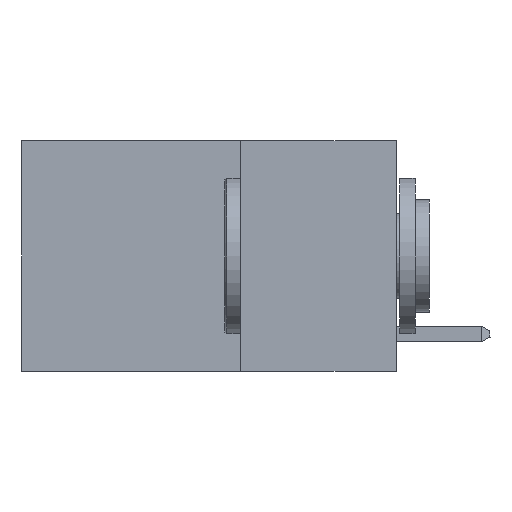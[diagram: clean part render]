
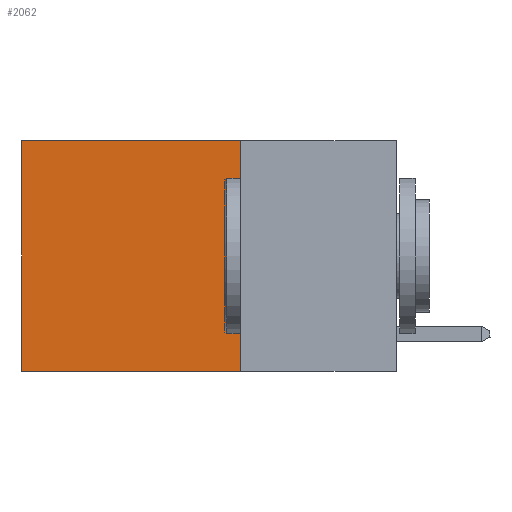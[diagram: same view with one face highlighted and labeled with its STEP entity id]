
A CAD part, left-side view. The second image highlights one B-rep face of the part: STEP entity #2062.
In plain terms, the highlighted planar face has unit normal (-1, 0, 0).
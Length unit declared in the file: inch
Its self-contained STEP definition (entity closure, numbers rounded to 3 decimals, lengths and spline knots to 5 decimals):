
#1244 = ORIENTED_EDGE ( 'NONE', *, *, #11885, .T. ) ;
#1545 = VECTOR ( 'NONE', #14747, 39.37008 ) ;
#1650 = DIRECTION ( 'NONE',  ( 0., 0., -1. ) ) ;
#1776 = CARTESIAN_POINT ( 'NONE',  ( 0.2625, 0.25, 0. ) ) ;
#2062 = ADVANCED_FACE ( 'NONE', ( #4222 ), #3379, .F. ) ;
#2165 = VERTEX_POINT ( 'NONE', #12706 ) ;
#2240 = EDGE_CURVE ( 'NONE', #9153, #14307, #15468, .T. ) ;
#2312 = DIRECTION ( 'NONE',  ( 1., 0., 0. ) ) ;
#2478 = DIRECTION ( 'NONE',  ( 0., 0., -1. ) ) ;
#2665 = LINE ( 'NONE', #5310, #6970 ) ;
#3100 = ORIENTED_EDGE ( 'NONE', *, *, #7772, .T. ) ;
#3379 = PLANE ( 'NONE',  #15404 ) ;
#3946 = ORIENTED_EDGE ( 'NONE', *, *, #2240, .F. ) ;
#4141 = CARTESIAN_POINT ( 'NONE',  ( 0.2625, 0.25, 0. ) ) ;
#4222 = FACE_OUTER_BOUND ( 'NONE', #15835, .T. ) ;
#5247 = CARTESIAN_POINT ( 'NONE',  ( 0.2625, 0.25, -0.37 ) ) ;
#5310 = CARTESIAN_POINT ( 'NONE',  ( 0.2625, 0.6, 0. ) ) ;
#6302 = VERTEX_POINT ( 'NONE', #1776 ) ;
#6707 = DIRECTION ( 'NONE',  ( 0., 1., 0. ) ) ;
#6970 = VECTOR ( 'NONE', #2478, 39.37008 ) ;
#7032 = CARTESIAN_POINT ( 'NONE',  ( 0.2625, 0.25, -0.37 ) ) ;
#7256 = CARTESIAN_POINT ( 'NONE',  ( 0.2625, 0.25, 0. ) ) ;
#7772 = EDGE_CURVE ( 'NONE', #6302, #2165, #15935, .T. ) ;
#8689 = DIRECTION ( 'NONE',  ( 0., 0., -1. ) ) ;
#8755 = VECTOR ( 'NONE', #6707, 39.37008 ) ;
#9116 = LINE ( 'NONE', #7256, #15828 ) ;
#9153 = VERTEX_POINT ( 'NONE', #5247 ) ;
#9398 = CARTESIAN_POINT ( 'NONE',  ( 0.2625, 0.25, 0. ) ) ;
#10150 = CARTESIAN_POINT ( 'NONE',  ( 0.2625, 0.6, -0.37 ) ) ;
#11885 = EDGE_CURVE ( 'NONE', #2165, #14307, #2665, .T. ) ;
#12706 = CARTESIAN_POINT ( 'NONE',  ( 0.2625, 0.6, 0. ) ) ;
#14274 = EDGE_CURVE ( 'NONE', #6302, #9153, #9116, .T. ) ;
#14307 = VERTEX_POINT ( 'NONE', #10150 ) ;
#14747 = DIRECTION ( 'NONE',  ( 0., 1., 0. ) ) ;
#15404 = AXIS2_PLACEMENT_3D ( 'NONE', #4141, #2312, #1650 ) ;
#15468 = LINE ( 'NONE', #7032, #8755 ) ;
#15828 = VECTOR ( 'NONE', #8689, 39.37008 ) ;
#15835 = EDGE_LOOP ( 'NONE', ( #1244, #3946, #17654, #3100 ) ) ;
#15935 = LINE ( 'NONE', #9398, #1545 ) ;
#17654 = ORIENTED_EDGE ( 'NONE', *, *, #14274, .F. ) ;
